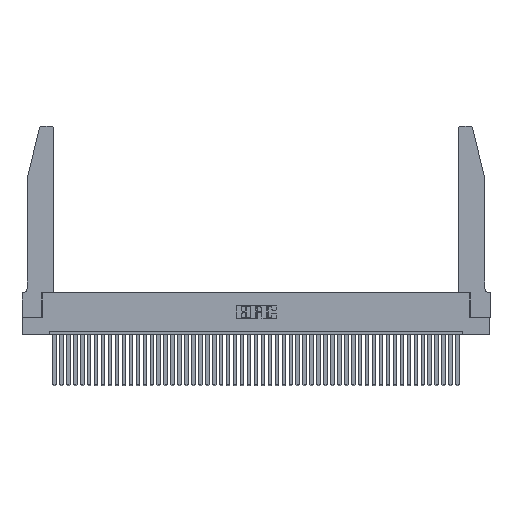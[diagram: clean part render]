
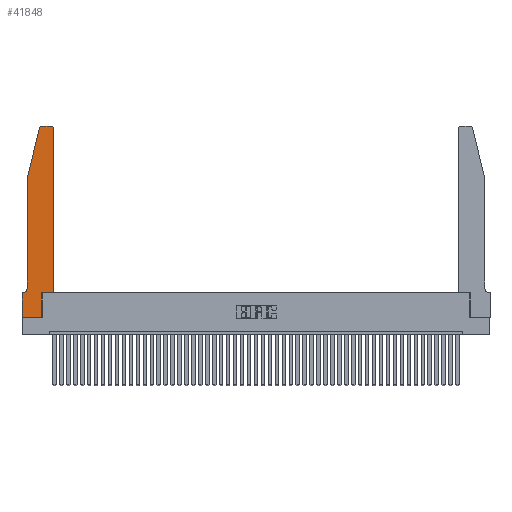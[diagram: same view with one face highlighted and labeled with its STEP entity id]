
A CAD part, top view. The second image highlights one B-rep face of the part: STEP entity #41848.
In plain terms, the highlighted planar face has unit normal (0, 0, 1).
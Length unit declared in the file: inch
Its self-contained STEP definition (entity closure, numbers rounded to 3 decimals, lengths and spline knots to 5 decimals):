
#1779 = CARTESIAN_POINT ( 'NONE',  ( 0., 0.35, 0.37 ) ) ;
#2041 = DIRECTION ( 'NONE',  ( 0., 1., 0. ) ) ;
#2394 = LINE ( 'NONE', #15299, #17036 ) ;
#2788 = DIRECTION ( 'NONE',  ( -1., 0., 0. ) ) ;
#2957 = CARTESIAN_POINT ( 'NONE',  ( 0., 0., 0.37 ) ) ;
#4340 = EDGE_CURVE ( 'NONE', #6993, #7272, #14995, .T. ) ;
#4869 = ORIENTED_EDGE ( 'NONE', *, *, #9280, .T. ) ;
#5119 = CARTESIAN_POINT ( 'NONE',  ( 0.0755, 0.35, 0.37 ) ) ;
#6050 = CARTESIAN_POINT ( 'NONE',  ( 0.0755, 0.42, 0.37 ) ) ;
#6168 = ORIENTED_EDGE ( 'NONE', *, *, #31172, .T. ) ;
#6474 = DIRECTION ( 'NONE',  ( -1., 0., 0. ) ) ;
#6923 = VERTEX_POINT ( 'NONE', #1779 ) ;
#6993 = VERTEX_POINT ( 'NONE', #12504 ) ;
#7218 = EDGE_CURVE ( 'NONE', #28256, #16049, #45686, .T. ) ;
#7272 = VERTEX_POINT ( 'NONE', #39689 ) ;
#8070 = AXIS2_PLACEMENT_3D ( 'NONE', #34731, #12851, #35055 ) ;
#8451 = ORIENTED_EDGE ( 'NONE', *, *, #46019, .T. ) ;
#8635 = CARTESIAN_POINT ( 'NONE',  ( 0.0055, 0.35, 0.37 ) ) ;
#9280 = EDGE_CURVE ( 'NONE', #30103, #6923, #26057, .T. ) ;
#10277 = VECTOR ( 'NONE', #35321, 39.37008 ) ;
#10319 = CARTESIAN_POINT ( 'NONE',  ( 0.0755, 2., 0.37 ) ) ;
#10900 = VECTOR ( 'NONE', #45835, 39.37008 ) ;
#11298 = ORIENTED_EDGE ( 'NONE', *, *, #36468, .T. ) ;
#12233 = CARTESIAN_POINT ( 'NONE',  ( 0.25487, 2.72718, 0.37 ) ) ;
#12452 = VERTEX_POINT ( 'NONE', #33341 ) ;
#12504 = CARTESIAN_POINT ( 'NONE',  ( 0.4205, 2.75, 0.37 ) ) ;
#12851 = DIRECTION ( 'NONE',  ( 0., 0., 1. ) ) ;
#13015 = PLANE ( 'NONE',  #8070 ) ;
#14454 = CARTESIAN_POINT ( 'NONE',  ( 0.4505, 0.35, 0.37 ) ) ;
#14995 = LINE ( 'NONE', #42330, #36356 ) ;
#15299 = CARTESIAN_POINT ( 'NONE',  ( 0.0755, 2., 0.37 ) ) ;
#15886 = CIRCLE ( 'NONE', #46501, 0.07 ) ;
#16049 = VERTEX_POINT ( 'NONE', #10319 ) ;
#16364 = CARTESIAN_POINT ( 'NONE',  ( 0.4205, 2.72, 0.37 ) ) ;
#16512 = DIRECTION ( 'NONE',  ( 0., 0., 1. ) ) ;
#17000 = VERTEX_POINT ( 'NONE', #40308 ) ;
#17036 = VECTOR ( 'NONE', #29746, 39.37008 ) ;
#17298 = DIRECTION ( 'NONE',  ( 0., 0., -1. ) ) ;
#17516 = CARTESIAN_POINT ( 'NONE',  ( 0.0755, 2., 0.37 ) ) ;
#17523 = CARTESIAN_POINT ( 'NONE',  ( 0., 0., 0.37 ) ) ;
#19830 = VECTOR ( 'NONE', #2041, 39.37008 ) ;
#21094 = ORIENTED_EDGE ( 'NONE', *, *, #4340, .T. ) ;
#23783 = ORIENTED_EDGE ( 'NONE', *, *, #36385, .T. ) ;
#24563 = CARTESIAN_POINT ( 'NONE',  ( 0.0055, 0.42, 0.37 ) ) ;
#24607 = LINE ( 'NONE', #14454, #45434 ) ;
#25580 = ORIENTED_EDGE ( 'NONE', *, *, #28113, .T. ) ;
#26057 = LINE ( 'NONE', #5119, #10900 ) ;
#26625 = FACE_OUTER_BOUND ( 'NONE', #28020, .T. ) ;
#27384 = ORIENTED_EDGE ( 'NONE', *, *, #46282, .T. ) ;
#27791 = EDGE_CURVE ( 'NONE', #28565, #17000, #29689, .T. ) ;
#28020 = EDGE_LOOP ( 'NONE', ( #21094, #8451, #28307, #23783, #35331, #4869, #38269, #6168, #36508, #25580, #11298, #27384 ) ) ;
#28113 = EDGE_CURVE ( 'NONE', #17000, #12452, #24607, .T. ) ;
#28256 = VERTEX_POINT ( 'NONE', #12233 ) ;
#28307 = ORIENTED_EDGE ( 'NONE', *, *, #7218, .T. ) ;
#28565 = VERTEX_POINT ( 'NONE', #35192 ) ;
#29689 = LINE ( 'NONE', #30065, #39246 ) ;
#29746 = DIRECTION ( 'NONE',  ( 0., -1., 0. ) ) ;
#30065 = CARTESIAN_POINT ( 'NONE',  ( 0.2865, 0.35, 0.37 ) ) ;
#30103 = VERTEX_POINT ( 'NONE', #8635 ) ;
#30373 = DIRECTION ( 'NONE',  ( 1., 0., 0. ) ) ;
#30384 = VERTEX_POINT ( 'NONE', #35726 ) ;
#31088 = LINE ( 'NONE', #38531, #19830 ) ;
#31172 = EDGE_CURVE ( 'NONE', #40696, #28565, #35573, .T. ) ;
#31948 = AXIS2_PLACEMENT_3D ( 'NONE', #37260, #33517, #30373 ) ;
#33168 = VERTEX_POINT ( 'NONE', #6050 ) ;
#33341 = CARTESIAN_POINT ( 'NONE',  ( 0.4505, 0.35, 0.37 ) ) ;
#33517 = DIRECTION ( 'NONE',  ( 0., 0., 1. ) ) ;
#33686 = DIRECTION ( 'NONE',  ( 0., 1., 0. ) ) ;
#34057 = LINE ( 'NONE', #39964, #43633 ) ;
#34731 = CARTESIAN_POINT ( 'NONE',  ( 0., 0.35, 0.37 ) ) ;
#34902 = EDGE_CURVE ( 'NONE', #6923, #40696, #34057, .T. ) ;
#35012 = VECTOR ( 'NONE', #42723, 39.37008 ) ;
#35055 = DIRECTION ( 'NONE',  ( 1., 0., 0. ) ) ;
#35192 = CARTESIAN_POINT ( 'NONE',  ( 0.2865, 0., 0.37 ) ) ;
#35321 = DIRECTION ( 'NONE',  ( -0.239, -0.971, 0. ) ) ;
#35331 = ORIENTED_EDGE ( 'NONE', *, *, #36547, .T. ) ;
#35573 = LINE ( 'NONE', #17523, #35012 ) ;
#35726 = CARTESIAN_POINT ( 'NONE',  ( 0.4505, 2.72, 0.37 ) ) ;
#36049 = CIRCLE ( 'NONE', #38265, 0.03 ) ;
#36356 = VECTOR ( 'NONE', #2788, 39.37008 ) ;
#36385 = EDGE_CURVE ( 'NONE', #16049, #33168, #2394, .T. ) ;
#36468 = EDGE_CURVE ( 'NONE', #12452, #30384, #31088, .T. ) ;
#36508 = ORIENTED_EDGE ( 'NONE', *, *, #27791, .T. ) ;
#36547 = EDGE_CURVE ( 'NONE', #33168, #30103, #15886, .T. ) ;
#36605 = DIRECTION ( 'NONE',  ( 1., 0., 0. ) ) ;
#37260 = CARTESIAN_POINT ( 'NONE',  ( 0.284, 2.72, 0.37 ) ) ;
#38265 = AXIS2_PLACEMENT_3D ( 'NONE', #16364, #16512, #45602 ) ;
#38269 = ORIENTED_EDGE ( 'NONE', *, *, #34902, .T. ) ;
#38531 = CARTESIAN_POINT ( 'NONE',  ( 0.4505, 0.35, 0.37 ) ) ;
#39209 = CIRCLE ( 'NONE', #31948, 0.03 ) ;
#39246 = VECTOR ( 'NONE', #33686, 39.37008 ) ;
#39689 = CARTESIAN_POINT ( 'NONE',  ( 0.284, 2.75, 0.37 ) ) ;
#39964 = CARTESIAN_POINT ( 'NONE',  ( 0., 0., 0.37 ) ) ;
#40308 = CARTESIAN_POINT ( 'NONE',  ( 0.2865, 0.35, 0.37 ) ) ;
#40435 = DIRECTION ( 'NONE',  ( 0., -1., 0. ) ) ;
#40696 = VERTEX_POINT ( 'NONE', #2957 ) ;
#41848 = ADVANCED_FACE ( 'NONE', ( #26625 ), #13015, .T. ) ;
#42330 = CARTESIAN_POINT ( 'NONE',  ( 0.2605, 2.75, 0.37 ) ) ;
#42723 = DIRECTION ( 'NONE',  ( 1., 0., 0. ) ) ;
#43633 = VECTOR ( 'NONE', #40435, 39.37008 ) ;
#45434 = VECTOR ( 'NONE', #36605, 39.37008 ) ;
#45602 = DIRECTION ( 'NONE',  ( 1., 0., 0. ) ) ;
#45686 = LINE ( 'NONE', #17516, #10277 ) ;
#45835 = DIRECTION ( 'NONE',  ( -1., 0., 0. ) ) ;
#46019 = EDGE_CURVE ( 'NONE', #7272, #28256, #39209, .T. ) ;
#46282 = EDGE_CURVE ( 'NONE', #30384, #6993, #36049, .T. ) ;
#46501 = AXIS2_PLACEMENT_3D ( 'NONE', #24563, #17298, #6474 ) ;
